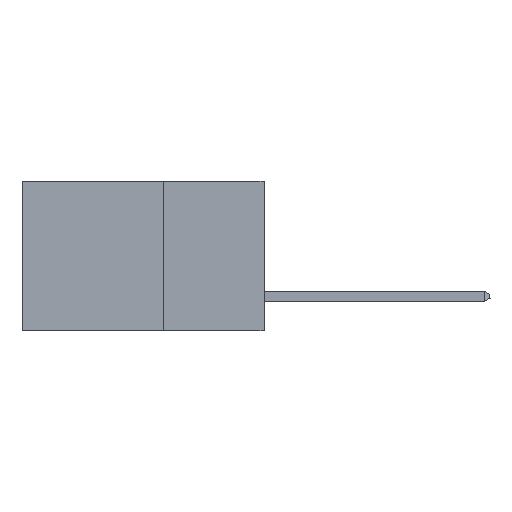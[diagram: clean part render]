
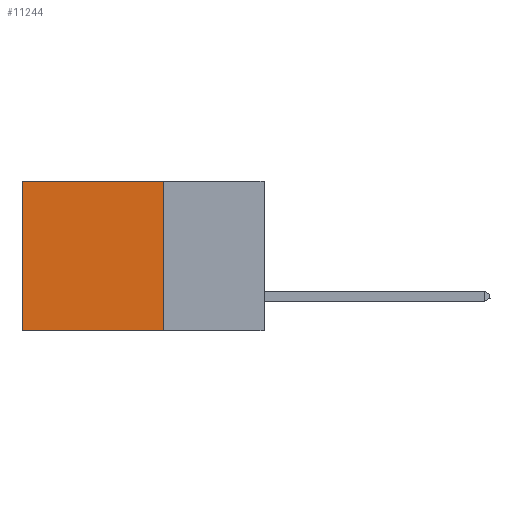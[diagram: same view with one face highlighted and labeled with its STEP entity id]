
A CAD part, left-side view. The second image highlights one B-rep face of the part: STEP entity #11244.
In plain terms, the highlighted planar face has unit normal (-1, 0, 0).
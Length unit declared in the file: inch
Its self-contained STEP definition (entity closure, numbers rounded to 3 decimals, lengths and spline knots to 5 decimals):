
#157 = EDGE_LOOP ( 'NONE', ( #9523, #9585, #10566, #9931 ) ) ;
#442 = CARTESIAN_POINT ( 'NONE',  ( 0.298, 0.25, 0. ) ) ;
#475 = EDGE_CURVE ( 'NONE', #2807, #2516, #4480, .T. ) ;
#599 = DIRECTION ( 'NONE',  ( 0., 0., -1. ) ) ;
#978 = CARTESIAN_POINT ( 'NONE',  ( 0.298, 0.6, 0. ) ) ;
#1548 = VECTOR ( 'NONE', #2778, 39.37008 ) ;
#1708 = CARTESIAN_POINT ( 'NONE',  ( 0.298, 0.25, -0.37 ) ) ;
#1805 = VECTOR ( 'NONE', #2383, 39.37008 ) ;
#2172 = VERTEX_POINT ( 'NONE', #10863 ) ;
#2383 = DIRECTION ( 'NONE',  ( 0., 0., -1. ) ) ;
#2516 = VERTEX_POINT ( 'NONE', #10274 ) ;
#2650 = EDGE_CURVE ( 'NONE', #9854, #2172, #3908, .T. ) ;
#2778 = DIRECTION ( 'NONE',  ( 0., 0., -1. ) ) ;
#2807 = VERTEX_POINT ( 'NONE', #5534 ) ;
#3323 = LINE ( 'NONE', #442, #8645 ) ;
#3908 = LINE ( 'NONE', #11302, #1805 ) ;
#4006 = EDGE_CURVE ( 'NONE', #9854, #2807, #3323, .T. ) ;
#4131 = DIRECTION ( 'NONE',  ( 0., 1., 0. ) ) ;
#4480 = LINE ( 'NONE', #978, #1548 ) ;
#4527 = LINE ( 'NONE', #1708, #9263 ) ;
#4950 = AXIS2_PLACEMENT_3D ( 'NONE', #5068, #11313, #599 ) ;
#5068 = CARTESIAN_POINT ( 'NONE',  ( 0.298, 0.25, 0. ) ) ;
#5320 = FACE_OUTER_BOUND ( 'NONE', #157, .T. ) ;
#5534 = CARTESIAN_POINT ( 'NONE',  ( 0.298, 0.6, 0. ) ) ;
#6038 = EDGE_CURVE ( 'NONE', #2172, #2516, #4527, .T. ) ;
#8645 = VECTOR ( 'NONE', #4131, 39.37008 ) ;
#9263 = VECTOR ( 'NONE', #10693, 39.37008 ) ;
#9523 = ORIENTED_EDGE ( 'NONE', *, *, #475, .T. ) ;
#9585 = ORIENTED_EDGE ( 'NONE', *, *, #6038, .F. ) ;
#9854 = VERTEX_POINT ( 'NONE', #11138 ) ;
#9931 = ORIENTED_EDGE ( 'NONE', *, *, #4006, .T. ) ;
#10274 = CARTESIAN_POINT ( 'NONE',  ( 0.298, 0.6, -0.37 ) ) ;
#10409 = PLANE ( 'NONE',  #4950 ) ;
#10566 = ORIENTED_EDGE ( 'NONE', *, *, #2650, .F. ) ;
#10693 = DIRECTION ( 'NONE',  ( 0., 1., 0. ) ) ;
#10863 = CARTESIAN_POINT ( 'NONE',  ( 0.298, 0.25, -0.37 ) ) ;
#11138 = CARTESIAN_POINT ( 'NONE',  ( 0.298, 0.25, 0. ) ) ;
#11244 = ADVANCED_FACE ( 'NONE', ( #5320 ), #10409, .F. ) ;
#11302 = CARTESIAN_POINT ( 'NONE',  ( 0.298, 0.25, 0. ) ) ;
#11313 = DIRECTION ( 'NONE',  ( 1., 0., 0. ) ) ;
